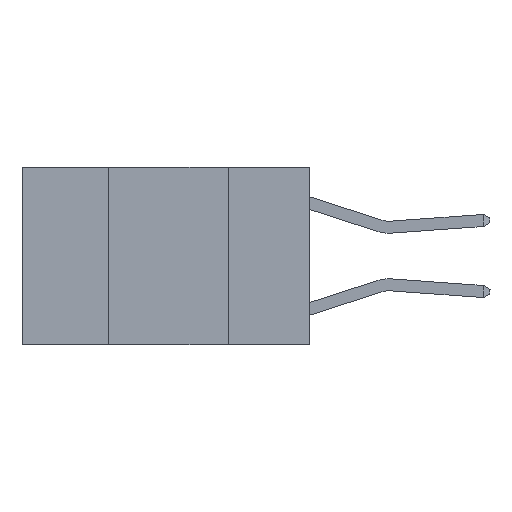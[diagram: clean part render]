
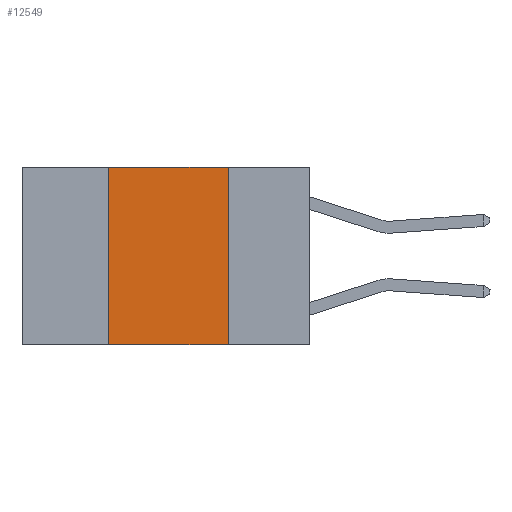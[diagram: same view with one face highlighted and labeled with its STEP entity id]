
A CAD part, left-side view. The second image highlights one B-rep face of the part: STEP entity #12549.
In plain terms, the highlighted planar face has unit normal (-1, 0, 0).
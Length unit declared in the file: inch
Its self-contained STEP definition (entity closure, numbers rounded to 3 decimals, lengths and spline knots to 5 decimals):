
#490 = DIRECTION ( 'NONE',  ( 0., -1., 0. ) ) ;
#826 = DIRECTION ( 'NONE',  ( 0., -1., 0. ) ) ;
#1245 = CARTESIAN_POINT ( 'NONE',  ( 0., 0.42, -0.37 ) ) ;
#1438 = CARTESIAN_POINT ( 'NONE',  ( 0., 0.42, 0. ) ) ;
#1776 = CARTESIAN_POINT ( 'NONE',  ( 0., 0.42, 0. ) ) ;
#2166 = LINE ( 'NONE', #12414, #13551 ) ;
#3116 = CARTESIAN_POINT ( 'NONE',  ( 0., 0.6, 0. ) ) ;
#3484 = VECTOR ( 'NONE', #9925, 39.37008 ) ;
#3821 = ORIENTED_EDGE ( 'NONE', *, *, #10598, .F. ) ;
#4215 = ORIENTED_EDGE ( 'NONE', *, *, #10284, .T. ) ;
#4509 = VERTEX_POINT ( 'NONE', #1438 ) ;
#4876 = DIRECTION ( 'NONE',  ( 1., 0., 0. ) ) ;
#5105 = VERTEX_POINT ( 'NONE', #8401 ) ;
#6026 = CARTESIAN_POINT ( 'NONE',  ( 0., 0.6, 0. ) ) ;
#6411 = EDGE_CURVE ( 'NONE', #4509, #8277, #10720, .T. ) ;
#6958 = EDGE_CURVE ( 'NONE', #9869, #4509, #12566, .T. ) ;
#7297 = CARTESIAN_POINT ( 'NONE',  ( 0., 0.17, 0. ) ) ;
#7476 = AXIS2_PLACEMENT_3D ( 'NONE', #6026, #4876, #12780 ) ;
#7981 = DIRECTION ( 'NONE',  ( 0., 0., -1. ) ) ;
#8028 = ORIENTED_EDGE ( 'NONE', *, *, #6411, .F. ) ;
#8064 = VECTOR ( 'NONE', #826, 39.37008 ) ;
#8277 = VERTEX_POINT ( 'NONE', #7297 ) ;
#8401 = CARTESIAN_POINT ( 'NONE',  ( 0., 0.17, -0.37 ) ) ;
#9532 = PLANE ( 'NONE',  #7476 ) ;
#9817 = CARTESIAN_POINT ( 'NONE',  ( 0., 0.6, -0.37 ) ) ;
#9869 = VERTEX_POINT ( 'NONE', #1245 ) ;
#9925 = DIRECTION ( 'NONE',  ( 0., 0., 1. ) ) ;
#10284 = EDGE_CURVE ( 'NONE', #9869, #5105, #13869, .T. ) ;
#10312 = ORIENTED_EDGE ( 'NONE', *, *, #6958, .F. ) ;
#10598 = EDGE_CURVE ( 'NONE', #8277, #5105, #2166, .T. ) ;
#10659 = VECTOR ( 'NONE', #490, 39.37008 ) ;
#10720 = LINE ( 'NONE', #3116, #8064 ) ;
#12414 = CARTESIAN_POINT ( 'NONE',  ( 0., 0.17, 0. ) ) ;
#12549 = ADVANCED_FACE ( 'NONE', ( #13336 ), #9532, .F. ) ;
#12566 = LINE ( 'NONE', #1776, #3484 ) ;
#12703 = EDGE_LOOP ( 'NONE', ( #3821, #8028, #10312, #4215 ) ) ;
#12780 = DIRECTION ( 'NONE',  ( 0., 0., -1. ) ) ;
#13336 = FACE_OUTER_BOUND ( 'NONE', #12703, .T. ) ;
#13551 = VECTOR ( 'NONE', #7981, 39.37008 ) ;
#13869 = LINE ( 'NONE', #9817, #10659 ) ;
